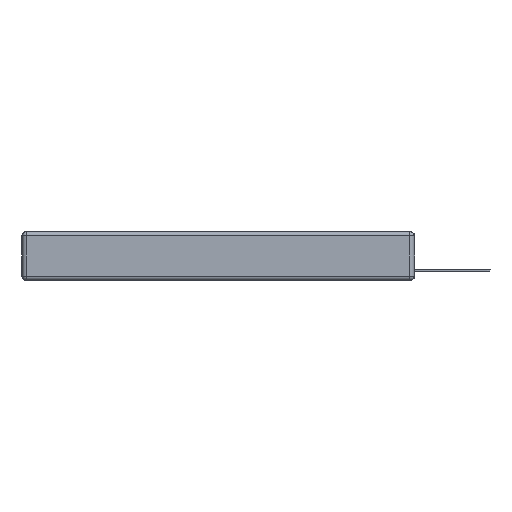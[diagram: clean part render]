
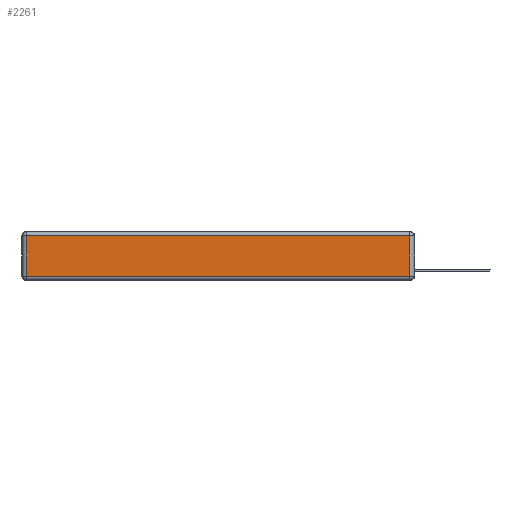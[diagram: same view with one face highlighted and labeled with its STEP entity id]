
A CAD part, left-side view. The second image highlights one B-rep face of the part: STEP entity #2261.
In plain terms, the highlighted planar face has unit normal (-1, 0, 0).
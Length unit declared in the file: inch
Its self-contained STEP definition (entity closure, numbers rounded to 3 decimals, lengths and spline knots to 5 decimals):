
#1904 = DIRECTION ( 'NONE',  ( 0., 0., -1. ) ) ;
#2261 = ADVANCED_FACE ( 'NONE', ( #17723 ), #5554, .T. ) ;
#2449 = VECTOR ( 'NONE', #5900, 39.37008 ) ;
#3676 = CARTESIAN_POINT ( 'NONE',  ( 0., 0.03, -0.03 ) ) ;
#4130 = CARTESIAN_POINT ( 'NONE',  ( 0., 2.72, -0.03 ) ) ;
#4489 = VERTEX_POINT ( 'NONE', #15746 ) ;
#5554 = PLANE ( 'NONE',  #15786 ) ;
#5660 = VECTOR ( 'NONE', #16775, 39.37008 ) ;
#5900 = DIRECTION ( 'NONE',  ( 0., 0., 1. ) ) ;
#6296 = VECTOR ( 'NONE', #14555, 39.37008 ) ;
#6315 = LINE ( 'NONE', #12010, #6567 ) ;
#6414 = ORIENTED_EDGE ( 'NONE', *, *, #15273, .T. ) ;
#6567 = VECTOR ( 'NONE', #1904, 39.37008 ) ;
#7183 = EDGE_CURVE ( 'NONE', #13271, #9596, #6315, .T. ) ;
#8243 = CARTESIAN_POINT ( 'NONE',  ( 0., 0., -0.313 ) ) ;
#8936 = CARTESIAN_POINT ( 'NONE',  ( 0., 2.72, -0.313 ) ) ;
#9053 = ORIENTED_EDGE ( 'NONE', *, *, #17547, .T. ) ;
#9223 = CARTESIAN_POINT ( 'NONE',  ( 0., 0.03, -0.343 ) ) ;
#9596 = VERTEX_POINT ( 'NONE', #8936 ) ;
#9609 = LINE ( 'NONE', #8243, #5660 ) ;
#10481 = CARTESIAN_POINT ( 'NONE',  ( 0., 0., -0.343 ) ) ;
#10627 = DIRECTION ( 'NONE',  ( 0., 0., 1. ) ) ;
#11007 = CARTESIAN_POINT ( 'NONE',  ( 0., 2.75, -0.03 ) ) ;
#12010 = CARTESIAN_POINT ( 'NONE',  ( 0., 2.72, -0.343 ) ) ;
#13271 = VERTEX_POINT ( 'NONE', #4130 ) ;
#13290 = LINE ( 'NONE', #9223, #2449 ) ;
#14317 = ORIENTED_EDGE ( 'NONE', *, *, #18332, .T. ) ;
#14475 = LINE ( 'NONE', #11007, #6296 ) ;
#14555 = DIRECTION ( 'NONE',  ( 0., 1., 0. ) ) ;
#15273 = EDGE_CURVE ( 'NONE', #19914, #13271, #14475, .T. ) ;
#15746 = CARTESIAN_POINT ( 'NONE',  ( 0., 0.03, -0.313 ) ) ;
#15786 = AXIS2_PLACEMENT_3D ( 'NONE', #10481, #19043, #10627 ) ;
#16775 = DIRECTION ( 'NONE',  ( 0., -1., 0. ) ) ;
#17547 = EDGE_CURVE ( 'NONE', #9596, #4489, #9609, .T. ) ;
#17723 = FACE_OUTER_BOUND ( 'NONE', #19433, .T. ) ;
#18332 = EDGE_CURVE ( 'NONE', #4489, #19914, #13290, .T. ) ;
#19043 = DIRECTION ( 'NONE',  ( -1., 0., 0. ) ) ;
#19433 = EDGE_LOOP ( 'NONE', ( #9053, #14317, #6414, #21777 ) ) ;
#19914 = VERTEX_POINT ( 'NONE', #3676 ) ;
#21777 = ORIENTED_EDGE ( 'NONE', *, *, #7183, .T. ) ;
